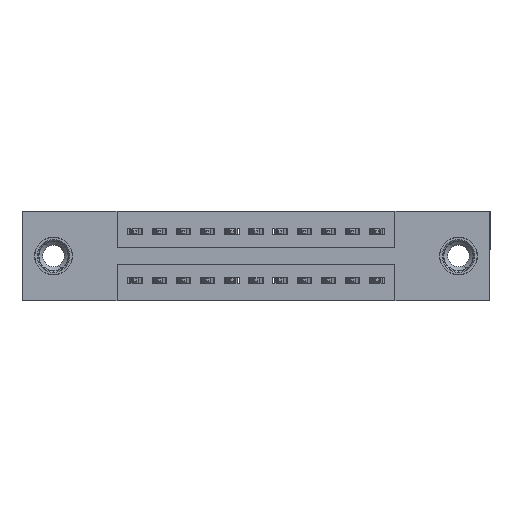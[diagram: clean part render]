
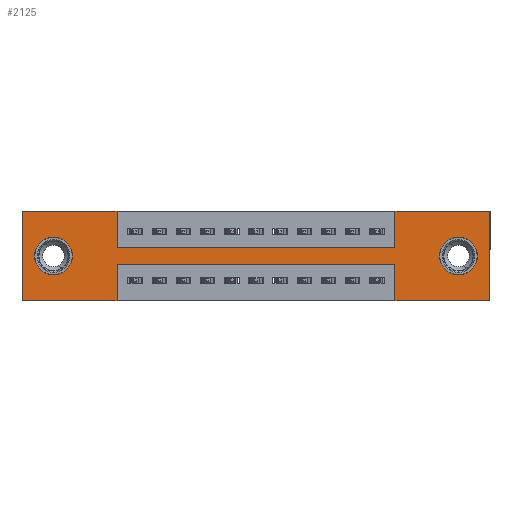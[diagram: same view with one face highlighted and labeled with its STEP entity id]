
A CAD part, front view. The second image highlights one B-rep face of the part: STEP entity #2125.
In plain terms, the highlighted planar face has unit normal (0, -1, 0).
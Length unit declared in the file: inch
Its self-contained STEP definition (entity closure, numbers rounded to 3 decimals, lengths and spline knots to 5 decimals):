
#194 = VERTEX_POINT ( 'NONE', #12353 ) ;
#225 = VERTEX_POINT ( 'NONE', #11862 ) ;
#358 = EDGE_CURVE ( 'NONE', #4279, #13010, #3191, .T. ) ;
#407 = DIRECTION ( 'NONE',  ( 0., 0., -1. ) ) ;
#499 = CARTESIAN_POINT ( 'NONE',  ( 1.5425, 0., -0.37 ) ) ;
#865 = EDGE_CURVE ( 'NONE', #14942, #225, #11794, .T. ) ;
#897 = VECTOR ( 'NONE', #3727, 39.37008 ) ;
#1251 = CARTESIAN_POINT ( 'NONE',  ( 1.5425, 0., 0. ) ) ;
#1278 = ORIENTED_EDGE ( 'NONE', *, *, #865, .F. ) ;
#1310 = LINE ( 'NONE', #6438, #10029 ) ;
#1345 = CARTESIAN_POINT ( 'NONE',  ( 1.5425, 0., -0.15 ) ) ;
#1470 = ORIENTED_EDGE ( 'NONE', *, *, #10342, .F. ) ;
#1671 = ORIENTED_EDGE ( 'NONE', *, *, #14128, .F. ) ;
#2125 = ADVANCED_FACE ( 'NONE', ( #13142, #7059, #4264 ), #10846, .T. ) ;
#2316 = CARTESIAN_POINT ( 'NONE',  ( 0., 0., -0.37 ) ) ;
#2323 = EDGE_CURVE ( 'NONE', #7539, #11667, #13620, .T. ) ;
#2534 = CARTESIAN_POINT ( 'NONE',  ( 1.5425, 0., 0. ) ) ;
#2601 = ORIENTED_EDGE ( 'NONE', *, *, #2323, .F. ) ;
#2792 = ORIENTED_EDGE ( 'NONE', *, *, #7966, .F. ) ;
#2816 = VERTEX_POINT ( 'NONE', #5630 ) ;
#2968 = VERTEX_POINT ( 'NONE', #2316 ) ;
#2982 = ORIENTED_EDGE ( 'NONE', *, *, #5810, .F. ) ;
#3191 = LINE ( 'NONE', #2534, #3964 ) ;
#3192 = CARTESIAN_POINT ( 'NONE',  ( 0.3925, 0., -0.15 ) ) ;
#3276 = DIRECTION ( 'NONE',  ( 0., 1., 0. ) ) ;
#3331 = VERTEX_POINT ( 'NONE', #499 ) ;
#3451 = DIRECTION ( 'NONE',  ( 0., 1., 0. ) ) ;
#3489 = CARTESIAN_POINT ( 'NONE',  ( 0., 0., -0.37 ) ) ;
#3490 = DIRECTION ( 'NONE',  ( 1., 0., 0. ) ) ;
#3637 = VECTOR ( 'NONE', #4575, 39.37008 ) ;
#3727 = DIRECTION ( 'NONE',  ( -1., 0., 0. ) ) ;
#3730 = ORIENTED_EDGE ( 'NONE', *, *, #10239, .T. ) ;
#3779 = CIRCLE ( 'NONE', #13608, 0.078 ) ;
#3885 = CARTESIAN_POINT ( 'NONE',  ( 0.3925, 0., -0.22 ) ) ;
#3964 = VECTOR ( 'NONE', #4753, 39.37008 ) ;
#3999 = LINE ( 'NONE', #12509, #9888 ) ;
#4264 = FACE_OUTER_BOUND ( 'NONE', #7124, .T. ) ;
#4279 = VERTEX_POINT ( 'NONE', #1345 ) ;
#4380 = LINE ( 'NONE', #3489, #3637 ) ;
#4442 = CARTESIAN_POINT ( 'NONE',  ( 0.3925, 0., 0. ) ) ;
#4575 = DIRECTION ( 'NONE',  ( -1., 0., 0. ) ) ;
#4685 = CARTESIAN_POINT ( 'NONE',  ( 0., 0., 0. ) ) ;
#4753 = DIRECTION ( 'NONE',  ( 0., 0., 1. ) ) ;
#4881 = CARTESIAN_POINT ( 'NONE',  ( 0., 0., 0. ) ) ;
#5240 = VECTOR ( 'NONE', #7607, 39.37008 ) ;
#5245 = CARTESIAN_POINT ( 'NONE',  ( 0., 0., 0. ) ) ;
#5447 = VECTOR ( 'NONE', #3490, 39.37008 ) ;
#5455 = DIRECTION ( 'NONE',  ( 0., 0., -1. ) ) ;
#5525 = DIRECTION ( 'NONE',  ( 0., 1., 0. ) ) ;
#5617 = VERTEX_POINT ( 'NONE', #4881 ) ;
#5630 = CARTESIAN_POINT ( 'NONE',  ( 0.13, 0., -0.107 ) ) ;
#5729 = DIRECTION ( 'NONE',  ( 0., 1., 0. ) ) ;
#5810 = EDGE_CURVE ( 'NONE', #5617, #7539, #10995, .T. ) ;
#6171 = ORIENTED_EDGE ( 'NONE', *, *, #6853, .F. ) ;
#6282 = EDGE_CURVE ( 'NONE', #6867, #7879, #14208, .T. ) ;
#6438 = CARTESIAN_POINT ( 'NONE',  ( 1.5425, 0., -0.37 ) ) ;
#6599 = CARTESIAN_POINT ( 'NONE',  ( 1.935, 0., 0. ) ) ;
#6853 = EDGE_CURVE ( 'NONE', #2968, #5617, #3999, .T. ) ;
#6867 = VERTEX_POINT ( 'NONE', #9103 ) ;
#6944 = CIRCLE ( 'NONE', #11403, 0.078 ) ;
#7059 = FACE_BOUND ( 'NONE', #8181, .T. ) ;
#7110 = CARTESIAN_POINT ( 'NONE',  ( 0.3925, 0., -0.37 ) ) ;
#7124 = EDGE_LOOP ( 'NONE', ( #10368, #1278, #2792, #10182, #13495, #1470, #8173, #11613, #2601, #2982, #6171, #1671 ) ) ;
#7132 = AXIS2_PLACEMENT_3D ( 'NONE', #7190, #11918, #11072 ) ;
#7190 = CARTESIAN_POINT ( 'NONE',  ( 0., 0., -0.37 ) ) ;
#7270 = LINE ( 'NONE', #9599, #897 ) ;
#7450 = CARTESIAN_POINT ( 'NONE',  ( 1.805, 0., -0.107 ) ) ;
#7536 = AXIS2_PLACEMENT_3D ( 'NONE', #12470, #5525, #13542 ) ;
#7539 = VERTEX_POINT ( 'NONE', #4442 ) ;
#7607 = DIRECTION ( 'NONE',  ( -1., 0., 0. ) ) ;
#7879 = VERTEX_POINT ( 'NONE', #7450 ) ;
#7966 = EDGE_CURVE ( 'NONE', #3331, #14942, #1310, .T. ) ;
#8173 = ORIENTED_EDGE ( 'NONE', *, *, #358, .F. ) ;
#8181 = EDGE_LOOP ( 'NONE', ( #9261, #3730 ) ) ;
#8261 = VECTOR ( 'NONE', #13300, 39.37008 ) ;
#8780 = EDGE_LOOP ( 'NONE', ( #14126, #14455 ) ) ;
#8921 = VECTOR ( 'NONE', #5455, 39.37008 ) ;
#9103 = CARTESIAN_POINT ( 'NONE',  ( 1.805, 0., -0.263 ) ) ;
#9135 = DIRECTION ( 'NONE',  ( 1., 0., 0. ) ) ;
#9261 = ORIENTED_EDGE ( 'NONE', *, *, #10109, .T. ) ;
#9362 = VERTEX_POINT ( 'NONE', #6599 ) ;
#9592 = CARTESIAN_POINT ( 'NONE',  ( 0.3925, 0., 0. ) ) ;
#9599 = CARTESIAN_POINT ( 'NONE',  ( 0., 0., -0.37 ) ) ;
#9878 = CARTESIAN_POINT ( 'NONE',  ( 0.13, 0., -0.263 ) ) ;
#9888 = VECTOR ( 'NONE', #10232, 39.37008 ) ;
#10029 = VECTOR ( 'NONE', #13288, 39.37008 ) ;
#10109 = EDGE_CURVE ( 'NONE', #2816, #10655, #11463, .T. ) ;
#10169 = CARTESIAN_POINT ( 'NONE',  ( 1.935, 0., 0. ) ) ;
#10182 = ORIENTED_EDGE ( 'NONE', *, *, #11102, .F. ) ;
#10193 = EDGE_CURVE ( 'NONE', #7879, #6867, #6944, .T. ) ;
#10232 = DIRECTION ( 'NONE',  ( 0., 0., 1. ) ) ;
#10239 = EDGE_CURVE ( 'NONE', #10655, #2816, #3779, .T. ) ;
#10256 = VECTOR ( 'NONE', #14564, 39.37008 ) ;
#10342 = EDGE_CURVE ( 'NONE', #13010, #9362, #14493, .T. ) ;
#10344 = CARTESIAN_POINT ( 'NONE',  ( 1.805, 0., -0.185 ) ) ;
#10368 = ORIENTED_EDGE ( 'NONE', *, *, #10792, .F. ) ;
#10505 = CARTESIAN_POINT ( 'NONE',  ( 1.805, 0., -0.185 ) ) ;
#10655 = VERTEX_POINT ( 'NONE', #9878 ) ;
#10686 = VECTOR ( 'NONE', #407, 39.37008 ) ;
#10792 = EDGE_CURVE ( 'NONE', #225, #11013, #14478, .T. ) ;
#10846 = PLANE ( 'NONE',  #7132 ) ;
#10995 = LINE ( 'NONE', #5245, #8261 ) ;
#11002 = AXIS2_PLACEMENT_3D ( 'NONE', #10505, #3451, #11639 ) ;
#11013 = VERTEX_POINT ( 'NONE', #7110 ) ;
#11072 = DIRECTION ( 'NONE',  ( 0., 0., -1. ) ) ;
#11102 = EDGE_CURVE ( 'NONE', #194, #3331, #7270, .T. ) ;
#11390 = EDGE_CURVE ( 'NONE', #11667, #4279, #14943, .T. ) ;
#11403 = AXIS2_PLACEMENT_3D ( 'NONE', #10344, #3276, #11480 ) ;
#11463 = CIRCLE ( 'NONE', #7536, 0.078 ) ;
#11480 = DIRECTION ( 'NONE',  ( 0., 0., -1. ) ) ;
#11613 = ORIENTED_EDGE ( 'NONE', *, *, #11390, .F. ) ;
#11639 = DIRECTION ( 'NONE',  ( 0., 0., -1. ) ) ;
#11667 = VERTEX_POINT ( 'NONE', #12957 ) ;
#11794 = LINE ( 'NONE', #3885, #5240 ) ;
#11862 = CARTESIAN_POINT ( 'NONE',  ( 0.3925, 0., -0.22 ) ) ;
#11918 = DIRECTION ( 'NONE',  ( 0., -1., 0. ) ) ;
#12353 = CARTESIAN_POINT ( 'NONE',  ( 1.935, 0., -0.37 ) ) ;
#12470 = CARTESIAN_POINT ( 'NONE',  ( 0.13, 0., -0.185 ) ) ;
#12487 = VECTOR ( 'NONE', #9135, 39.37008 ) ;
#12509 = CARTESIAN_POINT ( 'NONE',  ( 0., 0., 0. ) ) ;
#12669 = CARTESIAN_POINT ( 'NONE',  ( 0.13, 0., -0.185 ) ) ;
#12957 = CARTESIAN_POINT ( 'NONE',  ( 0.3925, 0., -0.15 ) ) ;
#13010 = VERTEX_POINT ( 'NONE', #1251 ) ;
#13142 = FACE_BOUND ( 'NONE', #8780, .T. ) ;
#13240 = LINE ( 'NONE', #10169, #10256 ) ;
#13288 = DIRECTION ( 'NONE',  ( 0., 0., 1. ) ) ;
#13300 = DIRECTION ( 'NONE',  ( 1., 0., 0. ) ) ;
#13483 = CARTESIAN_POINT ( 'NONE',  ( 0.3925, 0., -0.37 ) ) ;
#13495 = ORIENTED_EDGE ( 'NONE', *, *, #14518, .F. ) ;
#13542 = DIRECTION ( 'NONE',  ( 0., 0., 1. ) ) ;
#13608 = AXIS2_PLACEMENT_3D ( 'NONE', #12669, #5729, #13719 ) ;
#13620 = LINE ( 'NONE', #9592, #10686 ) ;
#13653 = CARTESIAN_POINT ( 'NONE',  ( 1.5425, 0., -0.22 ) ) ;
#13719 = DIRECTION ( 'NONE',  ( 0., 0., 1. ) ) ;
#14126 = ORIENTED_EDGE ( 'NONE', *, *, #10193, .T. ) ;
#14128 = EDGE_CURVE ( 'NONE', #11013, #2968, #4380, .T. ) ;
#14208 = CIRCLE ( 'NONE', #11002, 0.078 ) ;
#14455 = ORIENTED_EDGE ( 'NONE', *, *, #6282, .T. ) ;
#14478 = LINE ( 'NONE', #13483, #8921 ) ;
#14493 = LINE ( 'NONE', #4685, #5447 ) ;
#14518 = EDGE_CURVE ( 'NONE', #9362, #194, #13240, .T. ) ;
#14564 = DIRECTION ( 'NONE',  ( 0., 0., -1. ) ) ;
#14942 = VERTEX_POINT ( 'NONE', #13653 ) ;
#14943 = LINE ( 'NONE', #3192, #12487 ) ;
